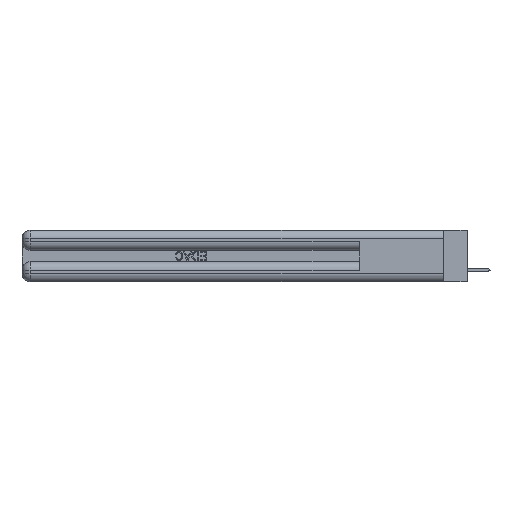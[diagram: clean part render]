
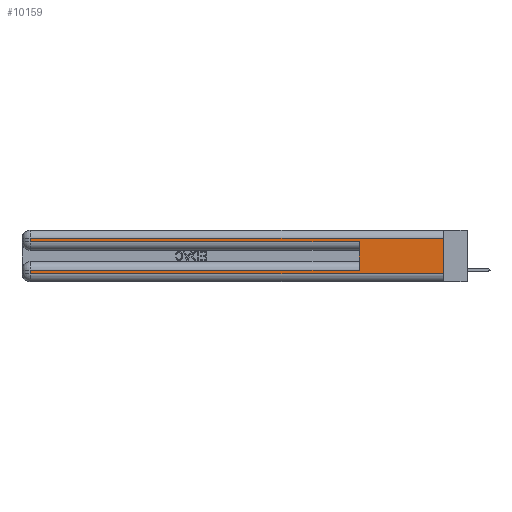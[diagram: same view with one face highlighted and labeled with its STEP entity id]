
A CAD part, left-side view. The second image highlights one B-rep face of the part: STEP entity #10159.
In plain terms, the highlighted planar face has unit normal (-1, 0, 0).
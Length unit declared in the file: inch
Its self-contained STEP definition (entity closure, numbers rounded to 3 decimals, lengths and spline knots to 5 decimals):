
#286 = AXIS2_PLACEMENT_3D ( 'NONE', #44899, #34304, #26793 ) ;
#768 = CARTESIAN_POINT ( 'NONE',  ( 0., 2.94, 0.37 ) ) ;
#1450 = CARTESIAN_POINT ( 'NONE',  ( 0., 0., 0.31 ) ) ;
#2551 = LINE ( 'NONE', #6737, #33283 ) ;
#2832 = CARTESIAN_POINT ( 'NONE',  ( 0., 0., 0.06 ) ) ;
#3633 = CARTESIAN_POINT ( 'NONE',  ( 0., 2.94, 0.285 ) ) ;
#5393 = LINE ( 'NONE', #41672, #41114 ) ;
#6737 = CARTESIAN_POINT ( 'NONE',  ( 0., 0.6, 0.145 ) ) ;
#8536 = VECTOR ( 'NONE', #38584, 39.37008 ) ;
#8908 = ORIENTED_EDGE ( 'NONE', *, *, #40899, .F. ) ;
#10029 = VERTEX_POINT ( 'NONE', #44527 ) ;
#10076 = EDGE_LOOP ( 'NONE', ( #44466, #33367, #25938, #10560, #8908, #20052, #13696, #32544 ) ) ;
#10159 = ADVANCED_FACE ( 'NONE', ( #16666 ), #30236, .F. ) ;
#10353 = EDGE_CURVE ( 'NONE', #17103, #42043, #41788, .T. ) ;
#10560 = ORIENTED_EDGE ( 'NONE', *, *, #28869, .T. ) ;
#11327 = EDGE_CURVE ( 'NONE', #21421, #12172, #15933, .T. ) ;
#11991 = DIRECTION ( 'NONE',  ( 0., -1., 0. ) ) ;
#12018 = VERTEX_POINT ( 'NONE', #27517 ) ;
#12172 = VERTEX_POINT ( 'NONE', #2832 ) ;
#13696 = ORIENTED_EDGE ( 'NONE', *, *, #28382, .T. ) ;
#13810 = LINE ( 'NONE', #33080, #23820 ) ;
#14705 = VECTOR ( 'NONE', #25488, 39.37008 ) ;
#14817 = DIRECTION ( 'NONE',  ( 0., 0., -1. ) ) ;
#15933 = LINE ( 'NONE', #29129, #35010 ) ;
#16666 = FACE_OUTER_BOUND ( 'NONE', #10076, .T. ) ;
#17103 = VERTEX_POINT ( 'NONE', #35059 ) ;
#18130 = EDGE_CURVE ( 'NONE', #34359, #10029, #5393, .T. ) ;
#18196 = VERTEX_POINT ( 'NONE', #3633 ) ;
#20052 = ORIENTED_EDGE ( 'NONE', *, *, #18130, .T. ) ;
#20437 = EDGE_CURVE ( 'NONE', #17103, #12172, #42066, .T. ) ;
#21421 = VERTEX_POINT ( 'NONE', #28330 ) ;
#22124 = CARTESIAN_POINT ( 'NONE',  ( 0., 0.6, 0.085 ) ) ;
#22758 = VECTOR ( 'NONE', #33338, 39.37008 ) ;
#22972 = CARTESIAN_POINT ( 'NONE',  ( 0., 2.94, 0.31 ) ) ;
#23820 = VECTOR ( 'NONE', #14817, 39.37008 ) ;
#25488 = DIRECTION ( 'NONE',  ( 0., 0., -1. ) ) ;
#25861 = LINE ( 'NONE', #768, #14705 ) ;
#25938 = ORIENTED_EDGE ( 'NONE', *, *, #30309, .T. ) ;
#26793 = DIRECTION ( 'NONE',  ( 0., 0., -1. ) ) ;
#27517 = CARTESIAN_POINT ( 'NONE',  ( 0., 0.6, 0.285 ) ) ;
#27732 = CARTESIAN_POINT ( 'NONE',  ( 0., 0., 0.285 ) ) ;
#28330 = CARTESIAN_POINT ( 'NONE',  ( 0., 2.94, 0.06 ) ) ;
#28382 = EDGE_CURVE ( 'NONE', #10029, #21421, #13810, .T. ) ;
#28869 = EDGE_CURVE ( 'NONE', #18196, #12018, #37183, .T. ) ;
#29129 = CARTESIAN_POINT ( 'NONE',  ( 0., 0., 0.06 ) ) ;
#30236 = PLANE ( 'NONE',  #286 ) ;
#30309 = EDGE_CURVE ( 'NONE', #42043, #18196, #25861, .T. ) ;
#32544 = ORIENTED_EDGE ( 'NONE', *, *, #11327, .T. ) ;
#33080 = CARTESIAN_POINT ( 'NONE',  ( 0., 2.94, 0.37 ) ) ;
#33283 = VECTOR ( 'NONE', #45749, 39.37008 ) ;
#33338 = DIRECTION ( 'NONE',  ( 0., 1., 0. ) ) ;
#33367 = ORIENTED_EDGE ( 'NONE', *, *, #10353, .T. ) ;
#34304 = DIRECTION ( 'NONE',  ( 1., 0., 0. ) ) ;
#34359 = VERTEX_POINT ( 'NONE', #22124 ) ;
#35010 = VECTOR ( 'NONE', #11991, 39.37008 ) ;
#35059 = CARTESIAN_POINT ( 'NONE',  ( 0., 0., 0.31 ) ) ;
#36077 = VECTOR ( 'NONE', #38203, 39.37008 ) ;
#37183 = LINE ( 'NONE', #27732, #36077 ) ;
#38203 = DIRECTION ( 'NONE',  ( 0., -1., 0. ) ) ;
#38584 = DIRECTION ( 'NONE',  ( 0., 0., -1. ) ) ;
#38657 = DIRECTION ( 'NONE',  ( 0., 1., 0. ) ) ;
#40899 = EDGE_CURVE ( 'NONE', #34359, #12018, #2551, .T. ) ;
#41114 = VECTOR ( 'NONE', #38657, 39.37008 ) ;
#41672 = CARTESIAN_POINT ( 'NONE',  ( 0., 0., 0.085 ) ) ;
#41788 = LINE ( 'NONE', #1450, #22758 ) ;
#42043 = VERTEX_POINT ( 'NONE', #22972 ) ;
#42066 = LINE ( 'NONE', #46066, #8536 ) ;
#44466 = ORIENTED_EDGE ( 'NONE', *, *, #20437, .F. ) ;
#44527 = CARTESIAN_POINT ( 'NONE',  ( 0., 2.94, 0.085 ) ) ;
#44899 = CARTESIAN_POINT ( 'NONE',  ( 0., 0., 0.37 ) ) ;
#45749 = DIRECTION ( 'NONE',  ( 0., 0., 1. ) ) ;
#46066 = CARTESIAN_POINT ( 'NONE',  ( 0., 0., 0.37 ) ) ;
